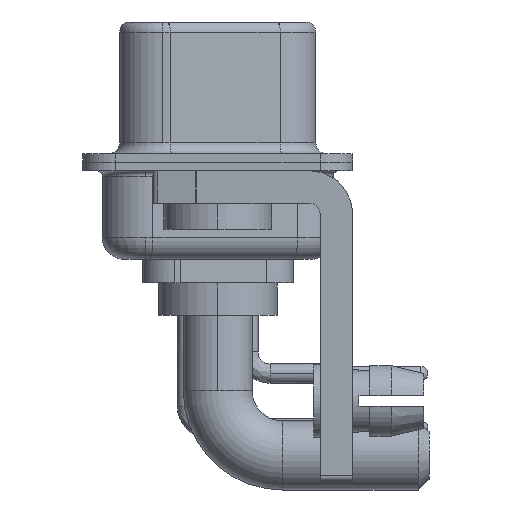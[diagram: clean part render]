
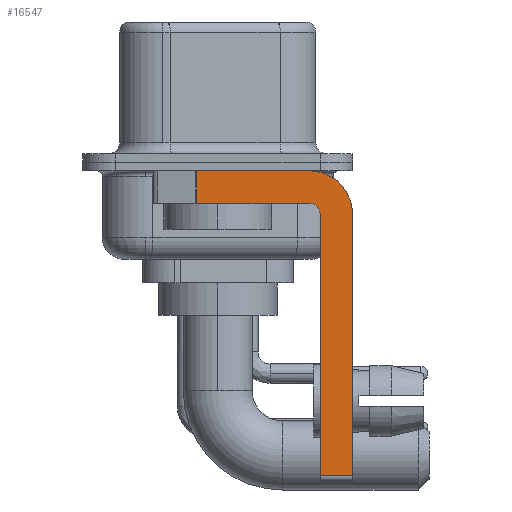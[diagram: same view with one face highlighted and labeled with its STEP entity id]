
A CAD part, left-side view. The second image highlights one B-rep face of the part: STEP entity #16547.
In plain terms, the highlighted planar face has unit normal (-1, 0, 0).
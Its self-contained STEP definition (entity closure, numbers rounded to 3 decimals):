
#54 = CARTESIAN_POINT ( 'NONE',  ( -2.9, -4.25, -2.4 ) ) ;
#1058 = CARTESIAN_POINT ( 'NONE',  ( -2.9, -4.25, -2.4 ) ) ;
#1158 = LINE ( 'NONE', #29494, #14005 ) ;
#1631 = DIRECTION ( 'NONE',  ( 1., 0., 0. ) ) ;
#1843 = VERTEX_POINT ( 'NONE', #21467 ) ;
#2900 = VERTEX_POINT ( 'NONE', #26970 ) ;
#3585 = VERTEX_POINT ( 'NONE', #6618 ) ;
#3988 = DIRECTION ( 'NONE',  ( 0., 0., -1. ) ) ;
#4235 = VERTEX_POINT ( 'NONE', #17782 ) ;
#4267 = VERTEX_POINT ( 'NONE', #5828 ) ;
#4768 = DIRECTION ( 'NONE',  ( 0., 0., 1. ) ) ;
#5465 = CARTESIAN_POINT ( 'NONE',  ( -2.9, 0.978, -1.9 ) ) ;
#5485 = DIRECTION ( 'NONE',  ( 0., 0., -1. ) ) ;
#5828 = CARTESIAN_POINT ( 'NONE',  ( -2.9, 0.978, -0.4 ) ) ;
#6201 = VERTEX_POINT ( 'NONE', #11756 ) ;
#6234 = ORIENTED_EDGE ( 'NONE', *, *, #24793, .F. ) ;
#6618 = CARTESIAN_POINT ( 'NONE',  ( -2.9, -4.75, -2.4 ) ) ;
#7469 = CARTESIAN_POINT ( 'NONE',  ( -2.9, -4.25, -0.4 ) ) ;
#7841 = ORIENTED_EDGE ( 'NONE', *, *, #8189, .F. ) ;
#8189 = EDGE_CURVE ( 'NONE', #11659, #23369, #19763, .T. ) ;
#8298 = VECTOR ( 'NONE', #11504, 1000. ) ;
#8459 = EDGE_CURVE ( 'NONE', #4267, #1843, #14669, .T. ) ;
#9792 = DIRECTION ( 'NONE',  ( 0., 0., -1. ) ) ;
#11504 = DIRECTION ( 'NONE',  ( 0., -1., 0. ) ) ;
#11517 = EDGE_CURVE ( 'NONE', #3585, #6201, #18504, .T. ) ;
#11541 = CARTESIAN_POINT ( 'NONE',  ( -2.9, -4.25, -1.9 ) ) ;
#11659 = VERTEX_POINT ( 'NONE', #7469 ) ;
#11756 = CARTESIAN_POINT ( 'NONE',  ( -2.9, -4.25, -1.9 ) ) ;
#12025 = ORIENTED_EDGE ( 'NONE', *, *, #8459, .T. ) ;
#14005 = VECTOR ( 'NONE', #22415, 1000. ) ;
#14519 = LINE ( 'NONE', #16857, #18391 ) ;
#14669 = LINE ( 'NONE', #5465, #16163 ) ;
#16163 = VECTOR ( 'NONE', #24659, 1000. ) ;
#16479 = ORIENTED_EDGE ( 'NONE', *, *, #11517, .F. ) ;
#16547 = ADVANCED_FACE ( 'NONE', ( #20832 ), #21143, .F. ) ;
#16857 = CARTESIAN_POINT ( 'NONE',  ( -2.9, -6.25, -2.4 ) ) ;
#16866 = LINE ( 'NONE', #11541, #28901 ) ;
#17021 = CARTESIAN_POINT ( 'NONE',  ( -2.9, -6.25, -2.4 ) ) ;
#17782 = CARTESIAN_POINT ( 'NONE',  ( -2.9, -4.75, -14.55 ) ) ;
#18054 = DIRECTION ( 'NONE',  ( 1., 0., 0. ) ) ;
#18391 = VECTOR ( 'NONE', #9792, 1000. ) ;
#18504 = CIRCLE ( 'NONE', #23546, 0.5 ) ;
#18998 = ORIENTED_EDGE ( 'NONE', *, *, #19040, .F. ) ;
#19040 = EDGE_CURVE ( 'NONE', #4235, #3585, #19745, .T. ) ;
#19745 = LINE ( 'NONE', #21803, #30487 ) ;
#19763 = CIRCLE ( 'NONE', #25289, 2. ) ;
#20832 = FACE_OUTER_BOUND ( 'NONE', #21243, .T. ) ;
#21112 = DIRECTION ( 'NONE',  ( 0., 1., 0. ) ) ;
#21143 = PLANE ( 'NONE',  #29413 ) ;
#21243 = EDGE_LOOP ( 'NONE', ( #30794, #12025, #23163, #16479, #18998, #26087, #6234, #7841 ) ) ;
#21467 = CARTESIAN_POINT ( 'NONE',  ( -2.9, 0.978, -1.9 ) ) ;
#21633 = EDGE_CURVE ( 'NONE', #6201, #1843, #16866, .T. ) ;
#21803 = CARTESIAN_POINT ( 'NONE',  ( -2.9, -4.75, -14.8 ) ) ;
#22415 = DIRECTION ( 'NONE',  ( 0., -1., 0. ) ) ;
#23163 = ORIENTED_EDGE ( 'NONE', *, *, #21633, .F. ) ;
#23369 = VERTEX_POINT ( 'NONE', #17021 ) ;
#23443 = CARTESIAN_POINT ( 'NONE',  ( -2.9, -4.25, -14.55 ) ) ;
#23546 = AXIS2_PLACEMENT_3D ( 'NONE', #54, #26183, #4768 ) ;
#23592 = EDGE_CURVE ( 'NONE', #4235, #2900, #25812, .T. ) ;
#24659 = DIRECTION ( 'NONE',  ( 0., 0., -1. ) ) ;
#24793 = EDGE_CURVE ( 'NONE', #23369, #2900, #14519, .T. ) ;
#25289 = AXIS2_PLACEMENT_3D ( 'NONE', #1058, #18054, #5485 ) ;
#25723 = CARTESIAN_POINT ( 'NONE',  ( -2.9, -4.25, -2.4 ) ) ;
#25812 = LINE ( 'NONE', #23443, #8298 ) ;
#26087 = ORIENTED_EDGE ( 'NONE', *, *, #23592, .T. ) ;
#26183 = DIRECTION ( 'NONE',  ( -1., 0., 0. ) ) ;
#26970 = CARTESIAN_POINT ( 'NONE',  ( -2.9, -6.25, -14.55 ) ) ;
#28873 = EDGE_CURVE ( 'NONE', #4267, #11659, #1158, .T. ) ;
#28879 = DIRECTION ( 'NONE',  ( 0., 0., 1. ) ) ;
#28901 = VECTOR ( 'NONE', #21112, 1000. ) ;
#29413 = AXIS2_PLACEMENT_3D ( 'NONE', #25723, #1631, #3988 ) ;
#29494 = CARTESIAN_POINT ( 'NONE',  ( -2.9, 3., -0.4 ) ) ;
#30487 = VECTOR ( 'NONE', #28879, 1000. ) ;
#30794 = ORIENTED_EDGE ( 'NONE', *, *, #28873, .F. ) ;
